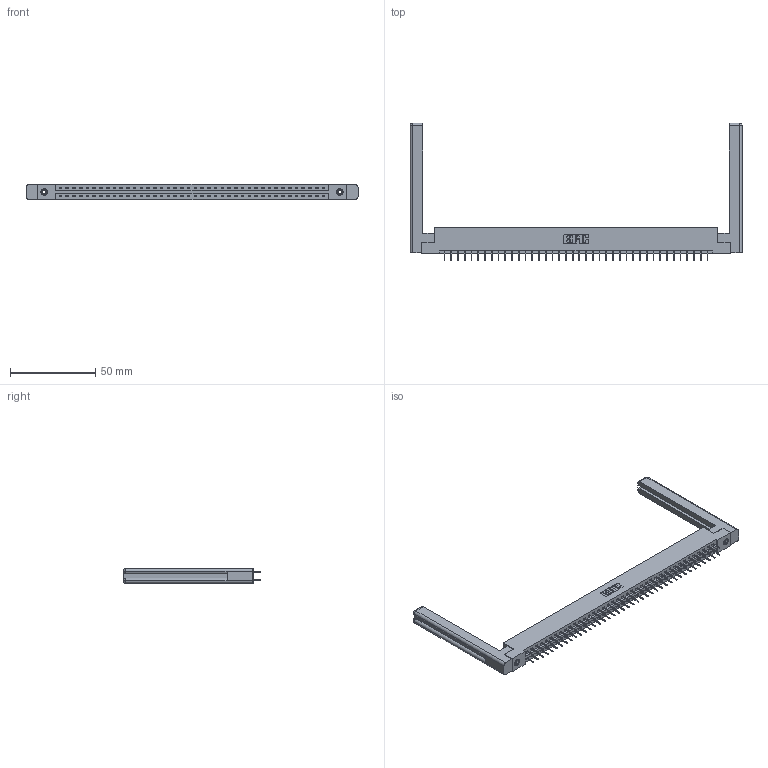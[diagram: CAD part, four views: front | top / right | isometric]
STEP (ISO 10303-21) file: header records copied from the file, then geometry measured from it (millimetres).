
FILE_DESCRIPTION (( 'STEP AP203' ), '1' );
FILE_NAME ('337-080-524-258.STEP', '2019-10-10T12:08:11', ( '' ), ( '' ), 'SwSTEP 2.0', 'SolidWorks 2016', '' );
FILE_SCHEMA (( 'CONFIG_CONTROL_DESIGN' ));
Length unit declared in the file: inch
Products named in the file (5): 307-220-058; 337 Part_Flush Mounting Lugs - 0.156 Dia-TI; 345-250-001_345-250-001-102; 345-292-001_345-293-124; 337-080-524-258
Assembly tree (85 placements, depth 2):
  337-080-524-258
    337 Part_Flush Mounting Lugs - 0.156 Dia-TI
    345-292-001_345-293-124  x80
    345-250-001_345-250-001-102  x2
    307-220-058  x2
Bounding box: 195.12 x 80.78 x 9.4 mm (x, y, z)
Volume: 27558.2 mm3; surface area: 27732.6 mm2
Topology: 85 solids, 85 shells, 4896 faces, 13865 edges, 8910 vertices
Faces by surface type: plane 3674, cylinder 1198, cone 12, torus 12
Entity records: 33980 total; most frequent: CARTESIAN_POINT 5733, ORIENTED_EDGE 5608, DIRECTION 4896, EDGE_CURVE 2804, VECTOR 2632, LINE 2632, VERTEX_POINT 1858, AXIS2_PLACEMENT_3D 1132
